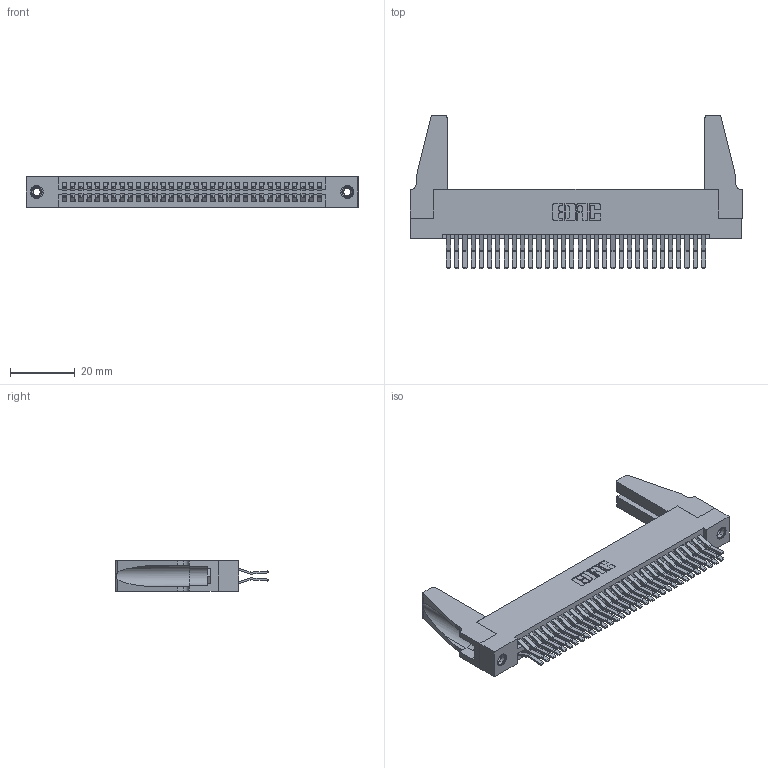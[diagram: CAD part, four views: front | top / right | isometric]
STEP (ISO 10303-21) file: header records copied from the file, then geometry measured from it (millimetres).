
FILE_DESCRIPTION (( 'STEP AP203' ), '1' );
FILE_NAME ('395-064-560-288.STEP', '2019-10-23T19:43:50', ( '' ), ( '' ), 'SwSTEP 2.0', 'SolidWorks 2016', '' );
FILE_SCHEMA (( 'CONFIG_CONTROL_DESIGN' ));
Length unit declared in the file: inch
Products named in the file (5): 345 Part_Flush Mounting Lugs - 0.156 Dia-TH; 345-292-001_560 Tail; 345-250-001_345-250-001-102; 345-220-078_345-220-088; 395-064-560-288
Assembly tree (69 placements, depth 2):
  395-064-560-288
    345 Part_Flush Mounting Lugs - 0.156 Dia-TH
    345-292-001_560 Tail  x64
    345-250-001_345-250-001-102  x2
    345-220-078_345-220-088  x2
Bounding box: 102.51 x 47.31 x 9.4 mm (x, y, z)
Volume: 13537.5 mm3; surface area: 19210.3 mm2
Topology: 69 solids, 69 shells, 3578 faces, 10575 edges, 6954 vertices
Faces by surface type: plane 2264, cylinder 1298, cone 12, torus 4
Entity records: 28690 total; most frequent: CARTESIAN_POINT 4814, ORIENTED_EDGE 4708, DIRECTION 4266, EDGE_CURVE 2354, LINE 2048, VECTOR 2048, VERTEX_POINT 1562, AXIS2_PLACEMENT_3D 1109
